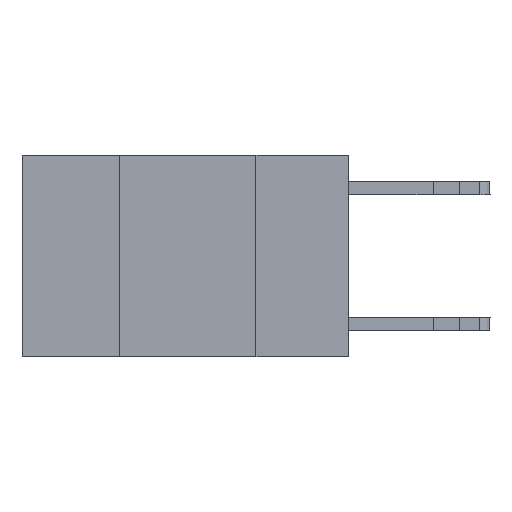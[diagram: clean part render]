
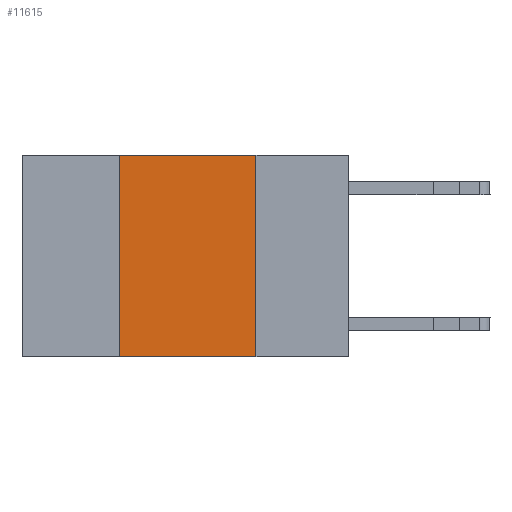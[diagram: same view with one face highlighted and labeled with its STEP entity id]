
A CAD part, left-side view. The second image highlights one B-rep face of the part: STEP entity #11615.
In plain terms, the highlighted planar face has unit normal (-1, 0, 0).
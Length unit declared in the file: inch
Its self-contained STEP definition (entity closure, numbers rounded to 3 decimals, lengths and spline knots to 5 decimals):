
#1172 = EDGE_CURVE ( 'NONE', #2545, #14289, #21324, .T. ) ;
#1769 = DIRECTION ( 'NONE',  ( 1., 0., 0. ) ) ;
#2470 = ORIENTED_EDGE ( 'NONE', *, *, #1172, .F. ) ;
#2545 = VERTEX_POINT ( 'NONE', #8870 ) ;
#2764 = CARTESIAN_POINT ( 'NONE',  ( 0., 0.17, -0.37 ) ) ;
#3419 = DIRECTION ( 'NONE',  ( 0., 0., -1. ) ) ;
#4851 = PLANE ( 'NONE',  #12287 ) ;
#4940 = CARTESIAN_POINT ( 'NONE',  ( 0., 0.42, 0. ) ) ;
#5301 = VECTOR ( 'NONE', #3419, 39.37008 ) ;
#5902 = DIRECTION ( 'NONE',  ( 0., -1., 0. ) ) ;
#7725 = DIRECTION ( 'NONE',  ( 0., -1., 0. ) ) ;
#8053 = EDGE_LOOP ( 'NONE', ( #13270, #10679, #2470, #21369 ) ) ;
#8140 = VECTOR ( 'NONE', #5902, 39.37008 ) ;
#8351 = DIRECTION ( 'NONE',  ( 0., 0., 1. ) ) ;
#8870 = CARTESIAN_POINT ( 'NONE',  ( 0., 0.42, -0.37 ) ) ;
#9731 = CARTESIAN_POINT ( 'NONE',  ( 0., 0.42, 0. ) ) ;
#10019 = DIRECTION ( 'NONE',  ( 0., 0., -1. ) ) ;
#10385 = EDGE_CURVE ( 'NONE', #2545, #21387, #15968, .T. ) ;
#10679 = ORIENTED_EDGE ( 'NONE', *, *, #13707, .F. ) ;
#11460 = CARTESIAN_POINT ( 'NONE',  ( 0., 0.6, 0. ) ) ;
#11615 = ADVANCED_FACE ( 'NONE', ( #16824 ), #4851, .F. ) ;
#12287 = AXIS2_PLACEMENT_3D ( 'NONE', #11460, #1769, #10019 ) ;
#12467 = CARTESIAN_POINT ( 'NONE',  ( 0., 0.6, -0.37 ) ) ;
#12903 = EDGE_CURVE ( 'NONE', #15999, #21387, #15086, .T. ) ;
#13270 = ORIENTED_EDGE ( 'NONE', *, *, #12903, .F. ) ;
#13707 = EDGE_CURVE ( 'NONE', #14289, #15999, #19416, .T. ) ;
#14289 = VERTEX_POINT ( 'NONE', #9731 ) ;
#15086 = LINE ( 'NONE', #16608, #5301 ) ;
#15968 = LINE ( 'NONE', #12467, #21110 ) ;
#15999 = VERTEX_POINT ( 'NONE', #16542 ) ;
#16127 = CARTESIAN_POINT ( 'NONE',  ( 0., 0.6, 0. ) ) ;
#16542 = CARTESIAN_POINT ( 'NONE',  ( 0., 0.17, 0. ) ) ;
#16608 = CARTESIAN_POINT ( 'NONE',  ( 0., 0.17, 0. ) ) ;
#16824 = FACE_OUTER_BOUND ( 'NONE', #8053, .T. ) ;
#19416 = LINE ( 'NONE', #16127, #8140 ) ;
#19777 = VECTOR ( 'NONE', #8351, 39.37008 ) ;
#21110 = VECTOR ( 'NONE', #7725, 39.37008 ) ;
#21324 = LINE ( 'NONE', #4940, #19777 ) ;
#21369 = ORIENTED_EDGE ( 'NONE', *, *, #10385, .T. ) ;
#21387 = VERTEX_POINT ( 'NONE', #2764 ) ;
